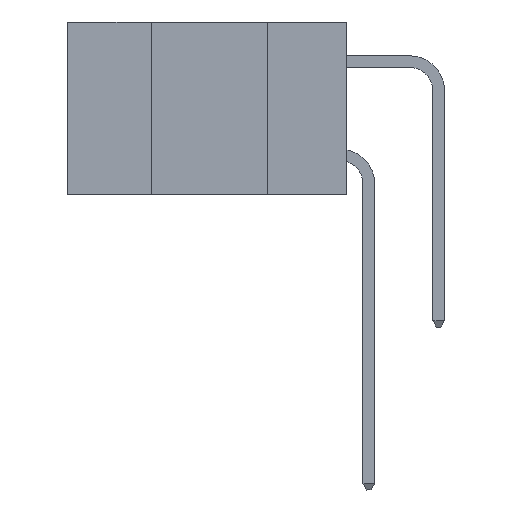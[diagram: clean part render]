
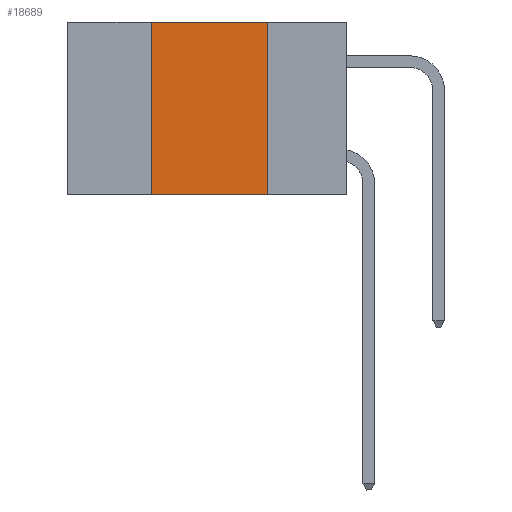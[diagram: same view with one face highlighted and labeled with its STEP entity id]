
A CAD part, left-side view. The second image highlights one B-rep face of the part: STEP entity #18689.
In plain terms, the highlighted planar face has unit normal (-1, 0, 0).
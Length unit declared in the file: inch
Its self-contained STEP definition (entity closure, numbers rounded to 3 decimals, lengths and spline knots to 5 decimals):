
#622 = CARTESIAN_POINT ( 'NONE',  ( 0., 0.42, 0. ) ) ;
#948 = VERTEX_POINT ( 'NONE', #12608 ) ;
#1039 = VERTEX_POINT ( 'NONE', #9643 ) ;
#1588 = VERTEX_POINT ( 'NONE', #13672 ) ;
#2250 = FACE_OUTER_BOUND ( 'NONE', #5556, .T. ) ;
#4477 = LINE ( 'NONE', #8041, #16547 ) ;
#4781 = DIRECTION ( 'NONE',  ( 0., -1., 0. ) ) ;
#5160 = CARTESIAN_POINT ( 'NONE',  ( 0., 0.17, 0. ) ) ;
#5288 = ORIENTED_EDGE ( 'NONE', *, *, #6573, .F. ) ;
#5556 = EDGE_LOOP ( 'NONE', ( #17773, #13313, #5288, #13493 ) ) ;
#5649 = AXIS2_PLACEMENT_3D ( 'NONE', #17389, #18886, #9853 ) ;
#6573 = EDGE_CURVE ( 'NONE', #1588, #7127, #18522, .T. ) ;
#6726 = DIRECTION ( 'NONE',  ( 0., 0., -1. ) ) ;
#6880 = PLANE ( 'NONE',  #5649 ) ;
#7127 = VERTEX_POINT ( 'NONE', #622 ) ;
#7544 = EDGE_CURVE ( 'NONE', #1588, #1039, #18693, .T. ) ;
#7818 = CARTESIAN_POINT ( 'NONE',  ( 0., 0.6, -0.37 ) ) ;
#8041 = CARTESIAN_POINT ( 'NONE',  ( 0., 0.6, 0. ) ) ;
#8558 = EDGE_CURVE ( 'NONE', #948, #1039, #16780, .T. ) ;
#9643 = CARTESIAN_POINT ( 'NONE',  ( 0., 0.17, -0.37 ) ) ;
#9853 = DIRECTION ( 'NONE',  ( 0., 0., -1. ) ) ;
#10014 = CARTESIAN_POINT ( 'NONE',  ( 0., 0.42, 0. ) ) ;
#10501 = VECTOR ( 'NONE', #11500, 39.37008 ) ;
#10696 = VECTOR ( 'NONE', #4781, 39.37008 ) ;
#11500 = DIRECTION ( 'NONE',  ( 0., 0., 1. ) ) ;
#12325 = VECTOR ( 'NONE', #6726, 39.37008 ) ;
#12336 = EDGE_CURVE ( 'NONE', #7127, #948, #4477, .T. ) ;
#12608 = CARTESIAN_POINT ( 'NONE',  ( 0., 0.17, 0. ) ) ;
#13313 = ORIENTED_EDGE ( 'NONE', *, *, #12336, .F. ) ;
#13493 = ORIENTED_EDGE ( 'NONE', *, *, #7544, .T. ) ;
#13672 = CARTESIAN_POINT ( 'NONE',  ( 0., 0.42, -0.37 ) ) ;
#16547 = VECTOR ( 'NONE', #18571, 39.37008 ) ;
#16780 = LINE ( 'NONE', #5160, #12325 ) ;
#17389 = CARTESIAN_POINT ( 'NONE',  ( 0., 0.6, 0. ) ) ;
#17773 = ORIENTED_EDGE ( 'NONE', *, *, #8558, .F. ) ;
#18522 = LINE ( 'NONE', #10014, #10501 ) ;
#18571 = DIRECTION ( 'NONE',  ( 0., -1., 0. ) ) ;
#18689 = ADVANCED_FACE ( 'NONE', ( #2250 ), #6880, .F. ) ;
#18693 = LINE ( 'NONE', #7818, #10696 ) ;
#18886 = DIRECTION ( 'NONE',  ( 1., 0., 0. ) ) ;
